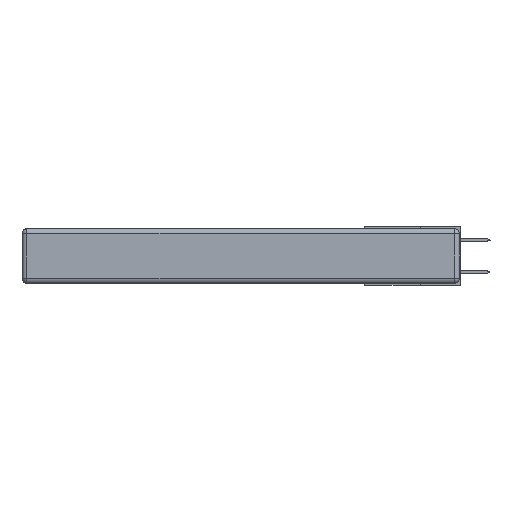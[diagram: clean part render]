
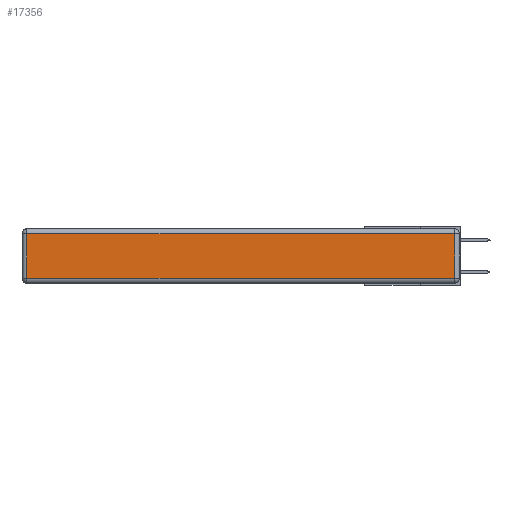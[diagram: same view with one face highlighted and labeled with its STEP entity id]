
A CAD part, left-side view. The second image highlights one B-rep face of the part: STEP entity #17356.
In plain terms, the highlighted planar face has unit normal (-1, 0, 0).
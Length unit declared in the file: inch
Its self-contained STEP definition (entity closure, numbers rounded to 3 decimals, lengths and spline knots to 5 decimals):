
#807 = VERTEX_POINT ( 'NONE', #8599 ) ;
#2287 = FACE_OUTER_BOUND ( 'NONE', #8614, .T. ) ;
#2520 = VECTOR ( 'NONE', #7925, 39.37008 ) ;
#2828 = EDGE_CURVE ( 'NONE', #16491, #4003, #4369, .T. ) ;
#3620 = CARTESIAN_POINT ( 'NONE',  ( 0., 2.72, -0.313 ) ) ;
#3804 = EDGE_CURVE ( 'NONE', #4778, #16491, #3868, .T. ) ;
#3868 = LINE ( 'NONE', #10958, #16441 ) ;
#4003 = VERTEX_POINT ( 'NONE', #3620 ) ;
#4225 = EDGE_CURVE ( 'NONE', #807, #4778, #8381, .T. ) ;
#4369 = LINE ( 'NONE', #5479, #5940 ) ;
#4382 = CARTESIAN_POINT ( 'NONE',  ( 0., 0., -0.313 ) ) ;
#4778 = VERTEX_POINT ( 'NONE', #9165 ) ;
#4810 = DIRECTION ( 'NONE',  ( -1., 0., 0. ) ) ;
#5479 = CARTESIAN_POINT ( 'NONE',  ( 0., 2.72, -0.343 ) ) ;
#5940 = VECTOR ( 'NONE', #15494, 39.37008 ) ;
#7231 = ORIENTED_EDGE ( 'NONE', *, *, #15267, .T. ) ;
#7925 = DIRECTION ( 'NONE',  ( 0., 0., 1. ) ) ;
#8381 = LINE ( 'NONE', #9377, #2520 ) ;
#8599 = CARTESIAN_POINT ( 'NONE',  ( 0., 0.03, -0.313 ) ) ;
#8614 = EDGE_LOOP ( 'NONE', ( #7231, #12541, #16072, #15351 ) ) ;
#9148 = CARTESIAN_POINT ( 'NONE',  ( 0., 0., -0.343 ) ) ;
#9165 = CARTESIAN_POINT ( 'NONE',  ( 0., 0.03, -0.03 ) ) ;
#9377 = CARTESIAN_POINT ( 'NONE',  ( 0., 0.03, -0.343 ) ) ;
#10593 = PLANE ( 'NONE',  #12517 ) ;
#10958 = CARTESIAN_POINT ( 'NONE',  ( 0., 2.75, -0.03 ) ) ;
#12392 = DIRECTION ( 'NONE',  ( 0., 1., 0. ) ) ;
#12517 = AXIS2_PLACEMENT_3D ( 'NONE', #9148, #4810, #13279 ) ;
#12541 = ORIENTED_EDGE ( 'NONE', *, *, #4225, .T. ) ;
#13279 = DIRECTION ( 'NONE',  ( 0., 0., 1. ) ) ;
#15267 = EDGE_CURVE ( 'NONE', #4003, #807, #17163, .T. ) ;
#15338 = VECTOR ( 'NONE', #18535, 39.37008 ) ;
#15351 = ORIENTED_EDGE ( 'NONE', *, *, #2828, .T. ) ;
#15494 = DIRECTION ( 'NONE',  ( 0., 0., -1. ) ) ;
#15890 = CARTESIAN_POINT ( 'NONE',  ( 0., 2.72, -0.03 ) ) ;
#16072 = ORIENTED_EDGE ( 'NONE', *, *, #3804, .T. ) ;
#16441 = VECTOR ( 'NONE', #12392, 39.37008 ) ;
#16491 = VERTEX_POINT ( 'NONE', #15890 ) ;
#17163 = LINE ( 'NONE', #4382, #15338 ) ;
#17356 = ADVANCED_FACE ( 'NONE', ( #2287 ), #10593, .T. ) ;
#18535 = DIRECTION ( 'NONE',  ( 0., -1., 0. ) ) ;
